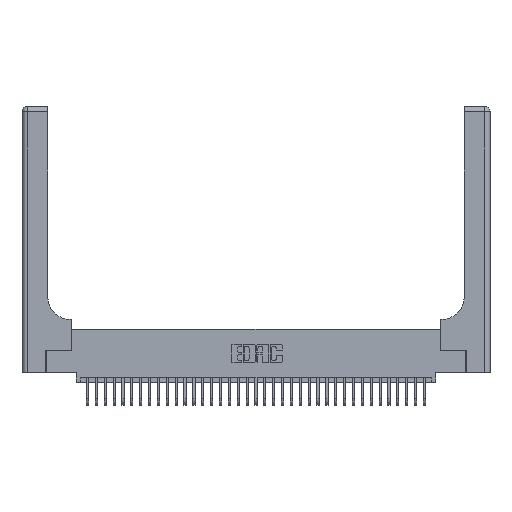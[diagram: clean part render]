
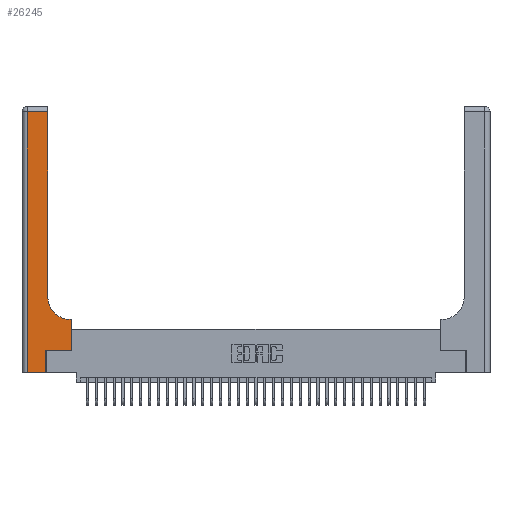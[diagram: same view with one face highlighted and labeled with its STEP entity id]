
A CAD part, top view. The second image highlights one B-rep face of the part: STEP entity #26245.
In plain terms, the highlighted planar face has unit normal (0, 0, 1).
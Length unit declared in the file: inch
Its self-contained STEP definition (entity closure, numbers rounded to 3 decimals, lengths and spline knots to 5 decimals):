
#565 = CARTESIAN_POINT ( 'NONE',  ( 0.5415, 0.85, 0.37 ) ) ;
#599 = ORIENTED_EDGE ( 'NONE', *, *, #24032, .T. ) ;
#1580 = VECTOR ( 'NONE', #17189, 39.37008 ) ;
#2109 = VECTOR ( 'NONE', #7398, 39.37008 ) ;
#2640 = VECTOR ( 'NONE', #35093, 39.37008 ) ;
#3284 = EDGE_LOOP ( 'NONE', ( #22257, #34946, #13843, #599, #30378, #33742, #29120, #34170, #15181 ) ) ;
#3312 = DIRECTION ( 'NONE',  ( 1., 0., 0. ) ) ;
#3999 = DIRECTION ( 'NONE',  ( 0., 1., 0. ) ) ;
#5523 = VECTOR ( 'NONE', #11715, 39.37008 ) ;
#5949 = CARTESIAN_POINT ( 'NONE',  ( 0., 3., 0.37 ) ) ;
#6126 = EDGE_CURVE ( 'NONE', #30819, #7405, #22971, .T. ) ;
#6199 = CARTESIAN_POINT ( 'NONE',  ( 0.2915, 3., 0.37 ) ) ;
#6743 = VERTEX_POINT ( 'NONE', #11174 ) ;
#6823 = CARTESIAN_POINT ( 'NONE',  ( 0.5585, 0.6, 0.37 ) ) ;
#7096 = LINE ( 'NONE', #12165, #27842 ) ;
#7322 = EDGE_CURVE ( 'NONE', #7405, #6743, #24067, .T. ) ;
#7372 = VERTEX_POINT ( 'NONE', #30530 ) ;
#7398 = DIRECTION ( 'NONE',  ( -1., 0., 0. ) ) ;
#7405 = VERTEX_POINT ( 'NONE', #9102 ) ;
#8123 = EDGE_CURVE ( 'NONE', #12967, #24590, #9210, .T. ) ;
#8948 = CARTESIAN_POINT ( 'NONE',  ( 0.269, 0.25, 0.37 ) ) ;
#9102 = CARTESIAN_POINT ( 'NONE',  ( 0.5415, 0.6, 0.37 ) ) ;
#9210 = LINE ( 'NONE', #20309, #14707 ) ;
#11174 = CARTESIAN_POINT ( 'NONE',  ( 0.2915, 0.85, 0.37 ) ) ;
#11482 = DIRECTION ( 'NONE',  ( -1., 0., 0. ) ) ;
#11715 = DIRECTION ( 'NONE',  ( 0., 1., 0. ) ) ;
#12077 = CARTESIAN_POINT ( 'NONE',  ( 0., 0., 0.37 ) ) ;
#12165 = CARTESIAN_POINT ( 'NONE',  ( 0., 2.94, 0.37 ) ) ;
#12967 = VERTEX_POINT ( 'NONE', #34948 ) ;
#13843 = ORIENTED_EDGE ( 'NONE', *, *, #25548, .T. ) ;
#13940 = PLANE ( 'NONE',  #19609 ) ;
#14025 = AXIS2_PLACEMENT_3D ( 'NONE', #565, #19636, #3312 ) ;
#14707 = VECTOR ( 'NONE', #3999, 39.37008 ) ;
#15181 = ORIENTED_EDGE ( 'NONE', *, *, #7322, .T. ) ;
#16980 = LINE ( 'NONE', #27896, #1580 ) ;
#17189 = DIRECTION ( 'NONE',  ( 0., 1., 0. ) ) ;
#17451 = EDGE_CURVE ( 'NONE', #6743, #7372, #33521, .T. ) ;
#17539 = DIRECTION ( 'NONE',  ( 1., 0., 0. ) ) ;
#18942 = CARTESIAN_POINT ( 'NONE',  ( 0.06, 3., 0.37 ) ) ;
#19609 = AXIS2_PLACEMENT_3D ( 'NONE', #5949, #27649, #11482 ) ;
#19636 = DIRECTION ( 'NONE',  ( 0., 0., -1. ) ) ;
#19913 = VECTOR ( 'NONE', #17539, 39.37008 ) ;
#20309 = CARTESIAN_POINT ( 'NONE',  ( 0.269, 0., 0.37 ) ) ;
#21912 = VERTEX_POINT ( 'NONE', #24356 ) ;
#22257 = ORIENTED_EDGE ( 'NONE', *, *, #17451, .T. ) ;
#22971 = LINE ( 'NONE', #26136, #2109 ) ;
#23029 = FACE_OUTER_BOUND ( 'NONE', #3284, .T. ) ;
#23914 = CARTESIAN_POINT ( 'NONE',  ( 0.06, 0., 0.37 ) ) ;
#23948 = EDGE_CURVE ( 'NONE', #21912, #30819, #16980, .T. ) ;
#24032 = EDGE_CURVE ( 'NONE', #30353, #12967, #27095, .T. ) ;
#24067 = CIRCLE ( 'NONE', #14025, 0.25 ) ;
#24344 = LINE ( 'NONE', #18942, #2640 ) ;
#24356 = CARTESIAN_POINT ( 'NONE',  ( 0.5585, 0.25, 0.37 ) ) ;
#24396 = CARTESIAN_POINT ( 'NONE',  ( 0.06, 2.94, 0.37 ) ) ;
#24590 = VERTEX_POINT ( 'NONE', #8948 ) ;
#24644 = CARTESIAN_POINT ( 'NONE',  ( 0.269, 0.25, 0.37 ) ) ;
#25548 = EDGE_CURVE ( 'NONE', #32247, #30353, #24344, .T. ) ;
#26136 = CARTESIAN_POINT ( 'NONE',  ( 0.2915, 0.6, 0.37 ) ) ;
#26245 = ADVANCED_FACE ( 'NONE', ( #23029 ), #13940, .F. ) ;
#27095 = LINE ( 'NONE', #12077, #19913 ) ;
#27356 = DIRECTION ( 'NONE',  ( 1., 0., 0. ) ) ;
#27649 = DIRECTION ( 'NONE',  ( 0., 0., -1. ) ) ;
#27842 = VECTOR ( 'NONE', #28362, 39.37008 ) ;
#27896 = CARTESIAN_POINT ( 'NONE',  ( 0.5585, 0.25, 0.37 ) ) ;
#28362 = DIRECTION ( 'NONE',  ( -1., 0., 0. ) ) ;
#28642 = LINE ( 'NONE', #24644, #34105 ) ;
#29120 = ORIENTED_EDGE ( 'NONE', *, *, #23948, .T. ) ;
#30353 = VERTEX_POINT ( 'NONE', #23914 ) ;
#30378 = ORIENTED_EDGE ( 'NONE', *, *, #8123, .T. ) ;
#30530 = CARTESIAN_POINT ( 'NONE',  ( 0.2915, 2.94, 0.37 ) ) ;
#30819 = VERTEX_POINT ( 'NONE', #6823 ) ;
#32247 = VERTEX_POINT ( 'NONE', #24396 ) ;
#33191 = EDGE_CURVE ( 'NONE', #7372, #32247, #7096, .T. ) ;
#33521 = LINE ( 'NONE', #6199, #5523 ) ;
#33742 = ORIENTED_EDGE ( 'NONE', *, *, #34043, .T. ) ;
#34043 = EDGE_CURVE ( 'NONE', #24590, #21912, #28642, .T. ) ;
#34105 = VECTOR ( 'NONE', #27356, 39.37008 ) ;
#34170 = ORIENTED_EDGE ( 'NONE', *, *, #6126, .T. ) ;
#34946 = ORIENTED_EDGE ( 'NONE', *, *, #33191, .T. ) ;
#34948 = CARTESIAN_POINT ( 'NONE',  ( 0.269, 0., 0.37 ) ) ;
#35093 = DIRECTION ( 'NONE',  ( 0., -1., 0. ) ) ;
